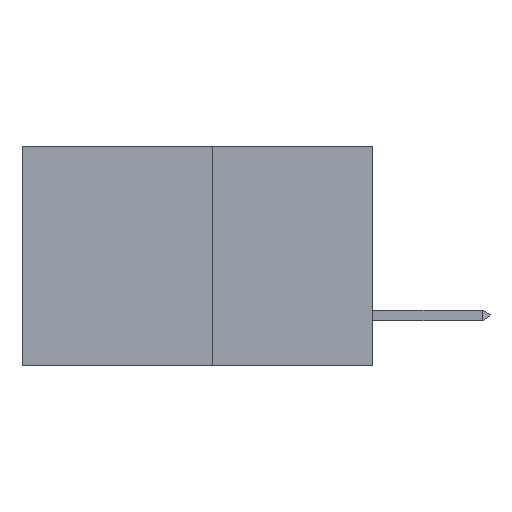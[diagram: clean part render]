
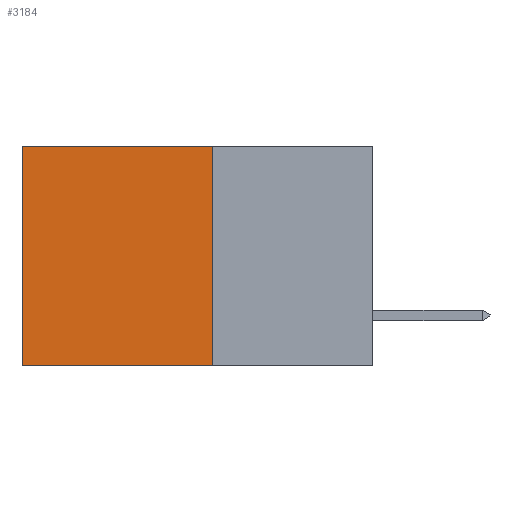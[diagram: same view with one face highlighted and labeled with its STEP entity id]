
A CAD part, left-side view. The second image highlights one B-rep face of the part: STEP entity #3184.
In plain terms, the highlighted planar face has unit normal (-1, 0, 0).
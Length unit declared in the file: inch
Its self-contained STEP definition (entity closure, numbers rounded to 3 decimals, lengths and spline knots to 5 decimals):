
#2547 = ORIENTED_EDGE ( 'NONE', *, *, #26827, .F. ) ;
#2787 = EDGE_LOOP ( 'NONE', ( #14859, #4597, #2547, #20129 ) ) ;
#3184 = ADVANCED_FACE ( 'NONE', ( #11530 ), #30305, .F. ) ;
#3602 = CARTESIAN_POINT ( 'NONE',  ( 0.277, 0.27, -0.37 ) ) ;
#3885 = EDGE_CURVE ( 'NONE', #29898, #22174, #22575, .T. ) ;
#4597 = ORIENTED_EDGE ( 'NONE', *, *, #11882, .F. ) ;
#7342 = VERTEX_POINT ( 'NONE', #30659 ) ;
#8785 = CARTESIAN_POINT ( 'NONE',  ( 0.277, 0.27, 0. ) ) ;
#8868 = LINE ( 'NONE', #25093, #23130 ) ;
#11530 = FACE_OUTER_BOUND ( 'NONE', #2787, .T. ) ;
#11798 = DIRECTION ( 'NONE',  ( 0., 1., 0. ) ) ;
#11882 = EDGE_CURVE ( 'NONE', #7342, #16143, #8868, .T. ) ;
#14354 = DIRECTION ( 'NONE',  ( 1., 0., 0. ) ) ;
#14491 = VECTOR ( 'NONE', #18104, 39.37008 ) ;
#14859 = ORIENTED_EDGE ( 'NONE', *, *, #24468, .T. ) ;
#16143 = VERTEX_POINT ( 'NONE', #29205 ) ;
#16262 = VECTOR ( 'NONE', #34358, 39.37008 ) ;
#18104 = DIRECTION ( 'NONE',  ( 0., 0., -1. ) ) ;
#20129 = ORIENTED_EDGE ( 'NONE', *, *, #3885, .T. ) ;
#22174 = VERTEX_POINT ( 'NONE', #29937 ) ;
#22442 = LINE ( 'NONE', #23368, #14491 ) ;
#22575 = LINE ( 'NONE', #32889, #28792 ) ;
#23130 = VECTOR ( 'NONE', #11798, 39.37008 ) ;
#23368 = CARTESIAN_POINT ( 'NONE',  ( 0.277, 0.27, -0.37 ) ) ;
#24468 = EDGE_CURVE ( 'NONE', #22174, #16143, #32055, .T. ) ;
#25093 = CARTESIAN_POINT ( 'NONE',  ( 0.277, 0.27, -0.37 ) ) ;
#26430 = CARTESIAN_POINT ( 'NONE',  ( 0.277, 0.59, -0.37 ) ) ;
#26827 = EDGE_CURVE ( 'NONE', #29898, #7342, #22442, .T. ) ;
#26873 = AXIS2_PLACEMENT_3D ( 'NONE', #3602, #14354, #32930 ) ;
#27593 = DIRECTION ( 'NONE',  ( 0., 1., 0. ) ) ;
#28792 = VECTOR ( 'NONE', #27593, 39.37008 ) ;
#29205 = CARTESIAN_POINT ( 'NONE',  ( 0.277, 0.59, -0.37 ) ) ;
#29898 = VERTEX_POINT ( 'NONE', #8785 ) ;
#29937 = CARTESIAN_POINT ( 'NONE',  ( 0.277, 0.59, 0. ) ) ;
#30305 = PLANE ( 'NONE',  #26873 ) ;
#30659 = CARTESIAN_POINT ( 'NONE',  ( 0.277, 0.27, -0.37 ) ) ;
#32055 = LINE ( 'NONE', #26430, #16262 ) ;
#32889 = CARTESIAN_POINT ( 'NONE',  ( 0.277, 0.27, 0. ) ) ;
#32930 = DIRECTION ( 'NONE',  ( 0., 0., -1. ) ) ;
#34358 = DIRECTION ( 'NONE',  ( 0., 0., -1. ) ) ;
